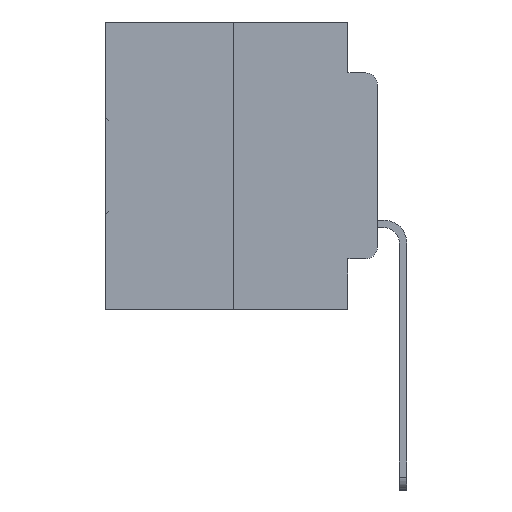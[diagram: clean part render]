
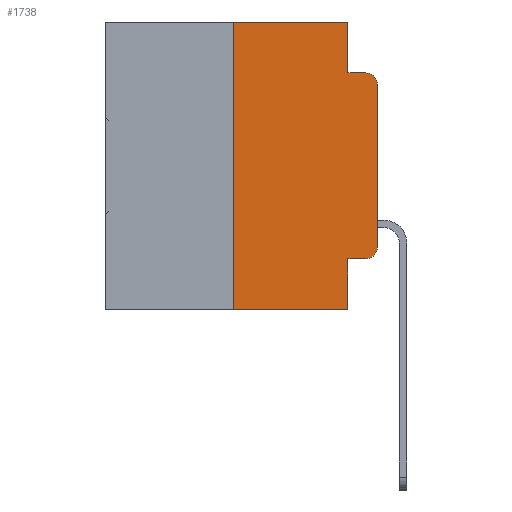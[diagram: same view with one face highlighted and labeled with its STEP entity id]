
A CAD part, left-side view. The second image highlights one B-rep face of the part: STEP entity #1738.
In plain terms, the highlighted planar face has unit normal (-1, 0, 0).
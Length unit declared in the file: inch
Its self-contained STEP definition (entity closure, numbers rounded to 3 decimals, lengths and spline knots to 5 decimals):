
#473 = DIRECTION ( 'NONE',  ( 0., -1., 0. ) ) ;
#790 = VERTEX_POINT ( 'NONE', #30387 ) ;
#987 = DIRECTION ( 'NONE',  ( -1., 0., 0. ) ) ;
#1671 = LINE ( 'NONE', #9329, #9088 ) ;
#1738 = ADVANCED_FACE ( 'NONE', ( #20585 ), #30843, .F. ) ;
#2060 = DIRECTION ( 'NONE',  ( 0., 0., -1. ) ) ;
#2233 = EDGE_CURVE ( 'NONE', #28129, #22664, #3020, .T. ) ;
#3020 = LINE ( 'NONE', #28261, #23366 ) ;
#4149 = VECTOR ( 'NONE', #11365, 39.37008 ) ;
#4808 = EDGE_CURVE ( 'NONE', #790, #29643, #33703, .T. ) ;
#5145 = VERTEX_POINT ( 'NONE', #15611 ) ;
#5909 = VECTOR ( 'NONE', #8712, 39.37008 ) ;
#6708 = VERTEX_POINT ( 'NONE', #23204 ) ;
#6733 = ORIENTED_EDGE ( 'NONE', *, *, #8228, .T. ) ;
#8228 = EDGE_CURVE ( 'NONE', #5145, #24489, #24340, .T. ) ;
#8712 = DIRECTION ( 'NONE',  ( 0., 0., -1. ) ) ;
#8957 = CARTESIAN_POINT ( 'NONE',  ( 0., 0.051, -0.4115 ) ) ;
#9088 = VECTOR ( 'NONE', #32590, 39.37008 ) ;
#9329 = CARTESIAN_POINT ( 'NONE',  ( 0., 0.051, 0. ) ) ;
#9745 = CARTESIAN_POINT ( 'NONE',  ( 0., 0.051, -0.0885 ) ) ;
#10000 = CARTESIAN_POINT ( 'NONE',  ( 0., 0.02, -0.3915 ) ) ;
#10250 = ORIENTED_EDGE ( 'NONE', *, *, #4808, .T. ) ;
#10933 = EDGE_CURVE ( 'NONE', #5145, #28129, #32813, .T. ) ;
#11008 = VECTOR ( 'NONE', #473, 39.37008 ) ;
#11365 = DIRECTION ( 'NONE',  ( 0., -1., 0. ) ) ;
#11415 = CARTESIAN_POINT ( 'NONE',  ( 0., 0.051, 0. ) ) ;
#12353 = VERTEX_POINT ( 'NONE', #26309 ) ;
#12586 = CIRCLE ( 'NONE', #15140, 0.02 ) ;
#12656 = DIRECTION ( 'NONE',  ( 0., 0., -1. ) ) ;
#13374 = EDGE_CURVE ( 'NONE', #6708, #790, #13765, .T. ) ;
#13501 = DIRECTION ( 'NONE',  ( 0., -1., 0. ) ) ;
#13765 = CIRCLE ( 'NONE', #30146, 0.02 ) ;
#14007 = CARTESIAN_POINT ( 'NONE',  ( 0., 0.473, -0.5 ) ) ;
#15140 = AXIS2_PLACEMENT_3D ( 'NONE', #17224, #987, #19863 ) ;
#15426 = ORIENTED_EDGE ( 'NONE', *, *, #16189, .F. ) ;
#15611 = CARTESIAN_POINT ( 'NONE',  ( 0., 0.25, -0.5 ) ) ;
#16069 = CARTESIAN_POINT ( 'NONE',  ( 0., 0.25, 0. ) ) ;
#16189 = EDGE_CURVE ( 'NONE', #22664, #18677, #27603, .T. ) ;
#16826 = CARTESIAN_POINT ( 'NONE',  ( 0., 0.25, 0. ) ) ;
#17109 = ORIENTED_EDGE ( 'NONE', *, *, #23772, .F. ) ;
#17224 = CARTESIAN_POINT ( 'NONE',  ( 0., 0.02, -0.1085 ) ) ;
#18051 = DIRECTION ( 'NONE',  ( 0., -1., 0. ) ) ;
#18196 = DIRECTION ( 'NONE',  ( 1., 0., 0. ) ) ;
#18229 = AXIS2_PLACEMENT_3D ( 'NONE', #33497, #18196, #2060 ) ;
#18677 = VERTEX_POINT ( 'NONE', #9745 ) ;
#19147 = ORIENTED_EDGE ( 'NONE', *, *, #10933, .F. ) ;
#19863 = DIRECTION ( 'NONE',  ( 0., 0., -1. ) ) ;
#20357 = EDGE_CURVE ( 'NONE', #12353, #6708, #31569, .T. ) ;
#20585 = FACE_OUTER_BOUND ( 'NONE', #23226, .T. ) ;
#20979 = CARTESIAN_POINT ( 'NONE',  ( 0., 0.02, -0.0885 ) ) ;
#22664 = VERTEX_POINT ( 'NONE', #32927 ) ;
#22797 = ORIENTED_EDGE ( 'NONE', *, *, #13374, .T. ) ;
#23123 = ORIENTED_EDGE ( 'NONE', *, *, #2233, .F. ) ;
#23204 = CARTESIAN_POINT ( 'NONE',  ( 0., 0.02, -0.4115 ) ) ;
#23226 = EDGE_LOOP ( 'NONE', ( #10250, #24238, #30285, #15426, #23123, #19147, #6733, #17109, #32341, #22797 ) ) ;
#23366 = VECTOR ( 'NONE', #18051, 39.37008 ) ;
#23772 = EDGE_CURVE ( 'NONE', #12353, #24489, #1671, .T. ) ;
#24112 = VERTEX_POINT ( 'NONE', #20979 ) ;
#24238 = ORIENTED_EDGE ( 'NONE', *, *, #31659, .T. ) ;
#24340 = LINE ( 'NONE', #14007, #4149 ) ;
#24489 = VERTEX_POINT ( 'NONE', #32424 ) ;
#26309 = CARTESIAN_POINT ( 'NONE',  ( 0., 0.051, -0.4115 ) ) ;
#26554 = EDGE_CURVE ( 'NONE', #18677, #24112, #28042, .T. ) ;
#26823 = VECTOR ( 'NONE', #33981, 39.37008 ) ;
#26940 = VECTOR ( 'NONE', #31680, 39.37008 ) ;
#27603 = LINE ( 'NONE', #11415, #5909 ) ;
#28042 = LINE ( 'NONE', #31473, #28821 ) ;
#28105 = DIRECTION ( 'NONE',  ( -1., 0., 0. ) ) ;
#28129 = VERTEX_POINT ( 'NONE', #16826 ) ;
#28261 = CARTESIAN_POINT ( 'NONE',  ( 0., 0.473, 0. ) ) ;
#28821 = VECTOR ( 'NONE', #13501, 39.37008 ) ;
#29122 = CARTESIAN_POINT ( 'NONE',  ( 0., 0., 0. ) ) ;
#29643 = VERTEX_POINT ( 'NONE', #32555 ) ;
#30146 = AXIS2_PLACEMENT_3D ( 'NONE', #10000, #28105, #12656 ) ;
#30285 = ORIENTED_EDGE ( 'NONE', *, *, #26554, .F. ) ;
#30387 = CARTESIAN_POINT ( 'NONE',  ( 0., 0., -0.3915 ) ) ;
#30843 = PLANE ( 'NONE',  #18229 ) ;
#31473 = CARTESIAN_POINT ( 'NONE',  ( 0., 0.051, -0.0885 ) ) ;
#31569 = LINE ( 'NONE', #8957, #11008 ) ;
#31659 = EDGE_CURVE ( 'NONE', #29643, #24112, #12586, .T. ) ;
#31680 = DIRECTION ( 'NONE',  ( 0., 0., 1. ) ) ;
#32341 = ORIENTED_EDGE ( 'NONE', *, *, #20357, .T. ) ;
#32424 = CARTESIAN_POINT ( 'NONE',  ( 0., 0.051, -0.5 ) ) ;
#32555 = CARTESIAN_POINT ( 'NONE',  ( 0., 0., -0.1085 ) ) ;
#32590 = DIRECTION ( 'NONE',  ( 0., 0., -1. ) ) ;
#32813 = LINE ( 'NONE', #16069, #26823 ) ;
#32927 = CARTESIAN_POINT ( 'NONE',  ( 0., 0.051, 0. ) ) ;
#33497 = CARTESIAN_POINT ( 'NONE',  ( 0., 0.473, 0. ) ) ;
#33703 = LINE ( 'NONE', #29122, #26940 ) ;
#33981 = DIRECTION ( 'NONE',  ( 0., 0., 1. ) ) ;
